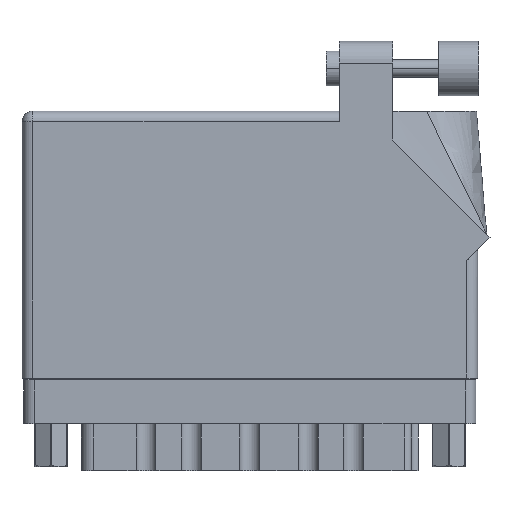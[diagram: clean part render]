
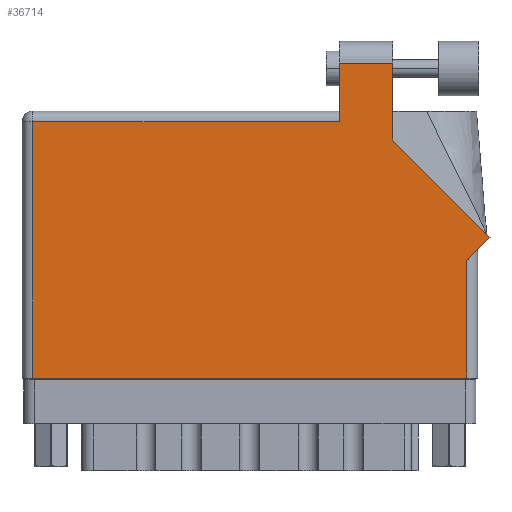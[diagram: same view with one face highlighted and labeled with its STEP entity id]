
A CAD part, front view. The second image highlights one B-rep face of the part: STEP entity #36714.
In plain terms, the highlighted face is planar.
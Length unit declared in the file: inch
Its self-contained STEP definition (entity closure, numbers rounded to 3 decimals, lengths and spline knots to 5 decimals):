
#211 = LINE ( 'NONE', #28084, #39355 ) ;
#1058 = VERTEX_POINT ( 'NONE', #24419 ) ;
#1803 = DIRECTION ( 'NONE',  ( 0., -1., 0. ) ) ;
#1837 = DIRECTION ( 'NONE',  ( 0., 1., 0. ) ) ;
#4153 = VERTEX_POINT ( 'NONE', #22748 ) ;
#4485 = VECTOR ( 'NONE', #59261, 39.37008 ) ;
#4679 = DIRECTION ( 'NONE',  ( 0., -1., 0. ) ) ;
#6599 = ORIENTED_EDGE ( 'NONE', *, *, #27117, .T. ) ;
#6946 = CARTESIAN_POINT ( 'NONE',  ( 2.126, 1.805, 0. ) ) ;
#6966 = ORIENTED_EDGE ( 'NONE', *, *, #20346, .T. ) ;
#7127 = CARTESIAN_POINT ( 'NONE',  ( 1.819, 1.805, 0. ) ) ;
#8880 = LINE ( 'NONE', #45984, #44286 ) ;
#9504 = DIRECTION ( 'NONE',  ( -1., 0., 0. ) ) ;
#10117 = CARTESIAN_POINT ( 'NONE',  ( 0., 1.53, 0. ) ) ;
#10237 = VERTEX_POINT ( 'NONE', #40270 ) ;
#11034 = ORIENTED_EDGE ( 'NONE', *, *, #52103, .T. ) ;
#13617 = LINE ( 'NONE', #49582, #4485 ) ;
#14357 = CARTESIAN_POINT ( 'NONE',  ( 2.55, 0., 0. ) ) ;
#14509 = VERTEX_POINT ( 'NONE', #29910 ) ;
#15302 = VERTEX_POINT ( 'NONE', #59277 ) ;
#15324 = EDGE_CURVE ( 'NONE', #1058, #16554, #52662, .T. ) ;
#16554 = VERTEX_POINT ( 'NONE', #6946 ) ;
#16762 = DIRECTION ( 'NONE',  ( 0.707, 0.707, 0. ) ) ;
#18634 = DIRECTION ( 'NONE',  ( 1., 0., 0. ) ) ;
#19333 = VERTEX_POINT ( 'NONE', #29702 ) ;
#19840 = DIRECTION ( 'NONE',  ( 0., 0., -1. ) ) ;
#20346 = EDGE_CURVE ( 'NONE', #15302, #37532, #51634, .T. ) ;
#22125 = EDGE_CURVE ( 'NONE', #10237, #4153, #211, .T. ) ;
#22748 = CARTESIAN_POINT ( 'NONE',  ( 1.819, 1.468, 0. ) ) ;
#22935 = ORIENTED_EDGE ( 'NONE', *, *, #39169, .T. ) ;
#24419 = CARTESIAN_POINT ( 'NONE',  ( 2.126, 1.36442, 0. ) ) ;
#25503 = CARTESIAN_POINT ( 'NONE',  ( 0., 1.468, 0. ) ) ;
#26733 = EDGE_LOOP ( 'NONE', ( #43476, #50952, #43795, #22935, #6599, #6966, #11034, #54941, #34879 ) ) ;
#26951 = CARTESIAN_POINT ( 'NONE',  ( 2.55, 0.737, 0. ) ) ;
#27108 = VECTOR ( 'NONE', #1837, 39.37008 ) ;
#27117 = EDGE_CURVE ( 'NONE', #55670, #15302, #42132, .T. ) ;
#28084 = CARTESIAN_POINT ( 'NONE',  ( 1.819, 1.53, 0. ) ) ;
#28480 = LINE ( 'NONE', #7127, #52544 ) ;
#29702 = CARTESIAN_POINT ( 'NONE',  ( 2.68271, 0.80771, 0. ) ) ;
#29910 = CARTESIAN_POINT ( 'NONE',  ( 2.55, 0.675, 0. ) ) ;
#30989 = CARTESIAN_POINT ( 'NONE',  ( 0.062, 1.468, 0. ) ) ;
#31778 = DIRECTION ( 'NONE',  ( 0., 1., 0. ) ) ;
#34879 = ORIENTED_EDGE ( 'NONE', *, *, #39647, .T. ) ;
#34925 = CARTESIAN_POINT ( 'NONE',  ( 2.126, 1.36442, 0. ) ) ;
#36714 = ADVANCED_FACE ( 'NONE', ( #42469 ), #57858, .F. ) ;
#37532 = VERTEX_POINT ( 'NONE', #14357 ) ;
#39169 = EDGE_CURVE ( 'NONE', #4153, #55670, #52717, .T. ) ;
#39355 = VECTOR ( 'NONE', #4679, 39.37008 ) ;
#39647 = EDGE_CURVE ( 'NONE', #19333, #1058, #13617, .T. ) ;
#39881 = VECTOR ( 'NONE', #1803, 39.37008 ) ;
#39972 = VECTOR ( 'NONE', #58702, 39.37008 ) ;
#40270 = CARTESIAN_POINT ( 'NONE',  ( 1.819, 1.805, 0. ) ) ;
#41024 = EDGE_CURVE ( 'NONE', #16554, #10237, #28480, .T. ) ;
#41055 = DIRECTION ( 'NONE',  ( -1., 0., 0. ) ) ;
#42132 = LINE ( 'NONE', #49773, #39881 ) ;
#42469 = FACE_OUTER_BOUND ( 'NONE', #26733, .T. ) ;
#43476 = ORIENTED_EDGE ( 'NONE', *, *, #15324, .T. ) ;
#43795 = ORIENTED_EDGE ( 'NONE', *, *, #22125, .T. ) ;
#44286 = VECTOR ( 'NONE', #16762, 39.37008 ) ;
#44596 = VECTOR ( 'NONE', #31778, 39.37008 ) ;
#44842 = AXIS2_PLACEMENT_3D ( 'NONE', #10117, #19840, #9504 ) ;
#45984 = CARTESIAN_POINT ( 'NONE',  ( 2.612, 0.737, 0. ) ) ;
#47426 = CARTESIAN_POINT ( 'NONE',  ( 0., 0., 0. ) ) ;
#49582 = CARTESIAN_POINT ( 'NONE',  ( 2.68271, 0.80771, 0. ) ) ;
#49773 = CARTESIAN_POINT ( 'NONE',  ( 0.062, 0., 0. ) ) ;
#50952 = ORIENTED_EDGE ( 'NONE', *, *, #41024, .T. ) ;
#51634 = LINE ( 'NONE', #47426, #58370 ) ;
#52103 = EDGE_CURVE ( 'NONE', #37532, #14509, #53544, .T. ) ;
#52544 = VECTOR ( 'NONE', #41055, 39.37008 ) ;
#52662 = LINE ( 'NONE', #34925, #27108 ) ;
#52717 = LINE ( 'NONE', #25503, #39972 ) ;
#53544 = LINE ( 'NONE', #26951, #44596 ) ;
#54941 = ORIENTED_EDGE ( 'NONE', *, *, #59671, .T. ) ;
#55670 = VERTEX_POINT ( 'NONE', #30989 ) ;
#57858 = PLANE ( 'NONE',  #44842 ) ;
#58370 = VECTOR ( 'NONE', #18634, 39.37008 ) ;
#58702 = DIRECTION ( 'NONE',  ( -1., 0., 0. ) ) ;
#59261 = DIRECTION ( 'NONE',  ( -0.707, 0.707, 0. ) ) ;
#59277 = CARTESIAN_POINT ( 'NONE',  ( 0.062, 0., 0. ) ) ;
#59671 = EDGE_CURVE ( 'NONE', #14509, #19333, #8880, .T. ) ;
